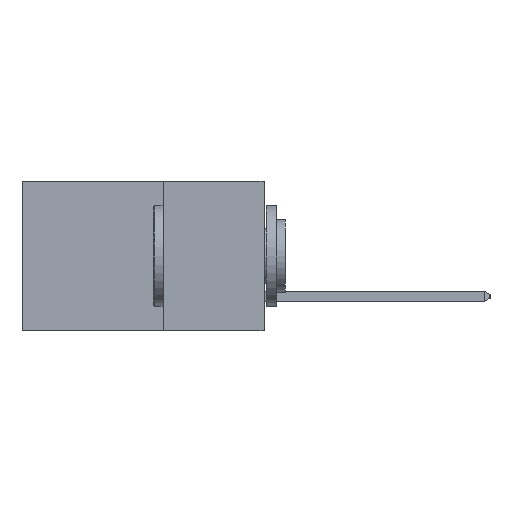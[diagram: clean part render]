
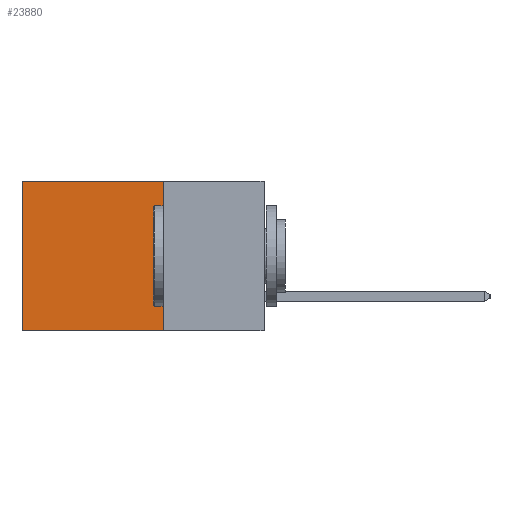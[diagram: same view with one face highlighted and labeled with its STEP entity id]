
A CAD part, left-side view. The second image highlights one B-rep face of the part: STEP entity #23880.
In plain terms, the highlighted planar face has unit normal (-1, 0, 0).
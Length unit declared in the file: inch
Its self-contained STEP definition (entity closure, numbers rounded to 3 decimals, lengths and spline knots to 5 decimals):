
#81 = LINE ( 'NONE', #12781, #779 ) ;
#779 = VECTOR ( 'NONE', #10672, 39.37008 ) ;
#1314 = VECTOR ( 'NONE', #15707, 39.37008 ) ;
#2141 = ORIENTED_EDGE ( 'NONE', *, *, #16537, .T. ) ;
#3242 = VERTEX_POINT ( 'NONE', #4023 ) ;
#4023 = CARTESIAN_POINT ( 'NONE',  ( 0.2615, 0.6, -0.37 ) ) ;
#4445 = PLANE ( 'NONE',  #26293 ) ;
#4764 = EDGE_CURVE ( 'NONE', #21706, #6739, #12188, .T. ) ;
#5497 = ORIENTED_EDGE ( 'NONE', *, *, #16974, .F. ) ;
#5621 = VECTOR ( 'NONE', #16145, 39.37008 ) ;
#5714 = CARTESIAN_POINT ( 'NONE',  ( 0.2615, 0.25, -0.37 ) ) ;
#6429 = ORIENTED_EDGE ( 'NONE', *, *, #4764, .F. ) ;
#6739 = VERTEX_POINT ( 'NONE', #5714 ) ;
#7522 = LINE ( 'NONE', #10062, #23423 ) ;
#8641 = DIRECTION ( 'NONE',  ( 0., 0., -1. ) ) ;
#9266 = EDGE_CURVE ( 'NONE', #21706, #12108, #81, .T. ) ;
#10062 = CARTESIAN_POINT ( 'NONE',  ( 0.2615, 0.6, -0.37 ) ) ;
#10672 = DIRECTION ( 'NONE',  ( 0., 1., 0. ) ) ;
#11433 = CARTESIAN_POINT ( 'NONE',  ( 0.2615, 0.25, -0.37 ) ) ;
#11866 = FACE_OUTER_BOUND ( 'NONE', #13849, .T. ) ;
#12108 = VERTEX_POINT ( 'NONE', #22475 ) ;
#12188 = LINE ( 'NONE', #16349, #5621 ) ;
#12781 = CARTESIAN_POINT ( 'NONE',  ( 0.2615, 0.25, 0. ) ) ;
#13556 = ORIENTED_EDGE ( 'NONE', *, *, #9266, .T. ) ;
#13849 = EDGE_LOOP ( 'NONE', ( #2141, #5497, #6429, #13556 ) ) ;
#15707 = DIRECTION ( 'NONE',  ( 0., 1., 0. ) ) ;
#16145 = DIRECTION ( 'NONE',  ( 0., 0., -1. ) ) ;
#16349 = CARTESIAN_POINT ( 'NONE',  ( 0.2615, 0.25, -0.37 ) ) ;
#16537 = EDGE_CURVE ( 'NONE', #12108, #3242, #7522, .T. ) ;
#16974 = EDGE_CURVE ( 'NONE', #6739, #3242, #23400, .T. ) ;
#19033 = CARTESIAN_POINT ( 'NONE',  ( 0.2615, 0.25, -0.37 ) ) ;
#21134 = DIRECTION ( 'NONE',  ( 1., 0., 0. ) ) ;
#21706 = VERTEX_POINT ( 'NONE', #25425 ) ;
#22475 = CARTESIAN_POINT ( 'NONE',  ( 0.2615, 0.6, 0. ) ) ;
#23400 = LINE ( 'NONE', #11433, #1314 ) ;
#23423 = VECTOR ( 'NONE', #24503, 39.37008 ) ;
#23880 = ADVANCED_FACE ( 'NONE', ( #11866 ), #4445, .F. ) ;
#24503 = DIRECTION ( 'NONE',  ( 0., 0., -1. ) ) ;
#25425 = CARTESIAN_POINT ( 'NONE',  ( 0.2615, 0.25, 0. ) ) ;
#26293 = AXIS2_PLACEMENT_3D ( 'NONE', #19033, #21134, #8641 ) ;
